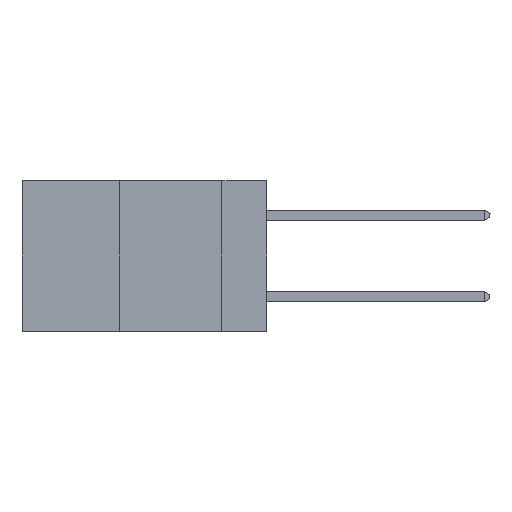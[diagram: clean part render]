
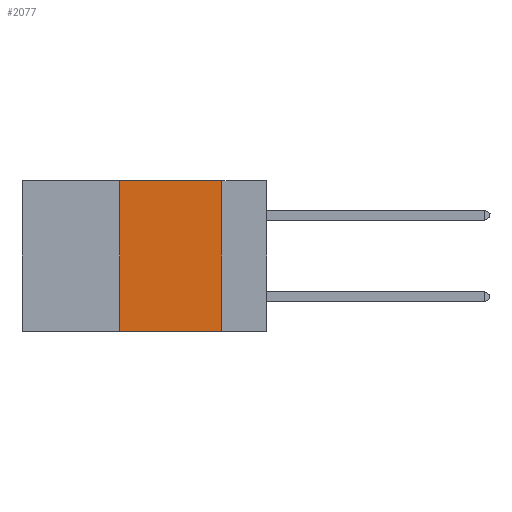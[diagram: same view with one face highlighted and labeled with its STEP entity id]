
A CAD part, left-side view. The second image highlights one B-rep face of the part: STEP entity #2077.
In plain terms, the highlighted planar face has unit normal (-1, 0, 0).
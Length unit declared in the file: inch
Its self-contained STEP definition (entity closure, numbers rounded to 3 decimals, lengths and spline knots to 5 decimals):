
#45 = CARTESIAN_POINT ( 'NONE',  ( 0., 0.6, 0. ) ) ;
#167 = VECTOR ( 'NONE', #13600, 39.37008 ) ;
#295 = CARTESIAN_POINT ( 'NONE',  ( 0., 0.36, 0. ) ) ;
#656 = LINE ( 'NONE', #45, #11660 ) ;
#1079 = ORIENTED_EDGE ( 'NONE', *, *, #12515, .T. ) ;
#1739 = ORIENTED_EDGE ( 'NONE', *, *, #11042, .F. ) ;
#1953 = VECTOR ( 'NONE', #12459, 39.37008 ) ;
#2077 = ADVANCED_FACE ( 'NONE', ( #5515 ), #10241, .F. ) ;
#2327 = LINE ( 'NONE', #11623, #13058 ) ;
#4188 = CARTESIAN_POINT ( 'NONE',  ( 0., 0.6, -0.37 ) ) ;
#4465 = VERTEX_POINT ( 'NONE', #10021 ) ;
#4584 = CARTESIAN_POINT ( 'NONE',  ( 0., 0.6, 0. ) ) ;
#4701 = ORIENTED_EDGE ( 'NONE', *, *, #11490, .F. ) ;
#5278 = EDGE_LOOP ( 'NONE', ( #1739, #12662, #4701, #1079 ) ) ;
#5515 = FACE_OUTER_BOUND ( 'NONE', #5278, .T. ) ;
#5760 = CARTESIAN_POINT ( 'NONE',  ( 0., 0.11, -0.37 ) ) ;
#6087 = LINE ( 'NONE', #9762, #167 ) ;
#7571 = VERTEX_POINT ( 'NONE', #7596 ) ;
#7596 = CARTESIAN_POINT ( 'NONE',  ( 0., 0.36, -0.37 ) ) ;
#7624 = EDGE_CURVE ( 'NONE', #9778, #4465, #656, .T. ) ;
#9647 = DIRECTION ( 'NONE',  ( 0., 0., 1. ) ) ;
#9688 = VERTEX_POINT ( 'NONE', #5760 ) ;
#9762 = CARTESIAN_POINT ( 'NONE',  ( 0., 0.11, 0. ) ) ;
#9778 = VERTEX_POINT ( 'NONE', #295 ) ;
#10021 = CARTESIAN_POINT ( 'NONE',  ( 0., 0.11, 0. ) ) ;
#10241 = PLANE ( 'NONE',  #10334 ) ;
#10334 = AXIS2_PLACEMENT_3D ( 'NONE', #4584, #10542, #10410 ) ;
#10410 = DIRECTION ( 'NONE',  ( 0., 0., -1. ) ) ;
#10542 = DIRECTION ( 'NONE',  ( 1., 0., 0. ) ) ;
#11042 = EDGE_CURVE ( 'NONE', #4465, #9688, #6087, .T. ) ;
#11490 = EDGE_CURVE ( 'NONE', #7571, #9778, #2327, .T. ) ;
#11623 = CARTESIAN_POINT ( 'NONE',  ( 0., 0.36, 0. ) ) ;
#11660 = VECTOR ( 'NONE', #12751, 39.37008 ) ;
#12459 = DIRECTION ( 'NONE',  ( 0., -1., 0. ) ) ;
#12515 = EDGE_CURVE ( 'NONE', #7571, #9688, #13036, .T. ) ;
#12662 = ORIENTED_EDGE ( 'NONE', *, *, #7624, .F. ) ;
#12751 = DIRECTION ( 'NONE',  ( 0., -1., 0. ) ) ;
#13036 = LINE ( 'NONE', #4188, #1953 ) ;
#13058 = VECTOR ( 'NONE', #9647, 39.37008 ) ;
#13600 = DIRECTION ( 'NONE',  ( 0., 0., -1. ) ) ;
